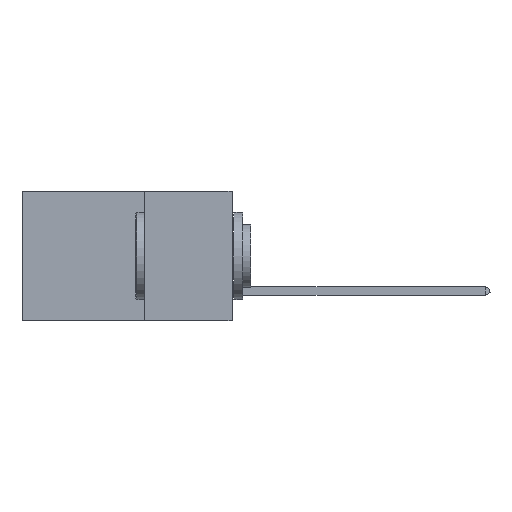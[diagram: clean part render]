
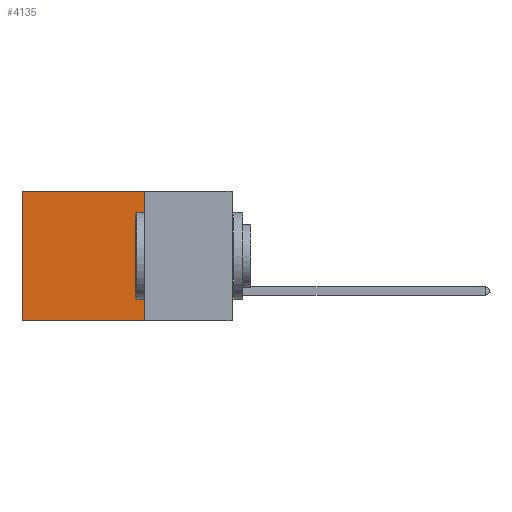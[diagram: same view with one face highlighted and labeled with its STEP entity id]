
A CAD part, left-side view. The second image highlights one B-rep face of the part: STEP entity #4135.
In plain terms, the highlighted planar face has unit normal (-1, 0, 0).
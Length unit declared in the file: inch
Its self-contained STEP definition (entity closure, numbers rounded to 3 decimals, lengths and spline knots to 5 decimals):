
#799 = CARTESIAN_POINT ( 'NONE',  ( 0.2875, 0.6, 0. ) ) ;
#937 = EDGE_CURVE ( 'NONE', #24279, #11036, #28548, .T. ) ;
#951 = LINE ( 'NONE', #27687, #5436 ) ;
#1014 = DIRECTION ( 'NONE',  ( 0., 1., 0. ) ) ;
#2587 = LINE ( 'NONE', #4025, #28113 ) ;
#3701 = EDGE_CURVE ( 'NONE', #27353, #11036, #27990, .T. ) ;
#4025 = CARTESIAN_POINT ( 'NONE',  ( 0.2875, 0.25, 0. ) ) ;
#4135 = ADVANCED_FACE ( 'NONE', ( #23472 ), #27661, .F. ) ;
#5126 = CARTESIAN_POINT ( 'NONE',  ( 0.2875, 0.25, -0.37 ) ) ;
#5436 = VECTOR ( 'NONE', #1014, 39.37008 ) ;
#5672 = ORIENTED_EDGE ( 'NONE', *, *, #3701, .T. ) ;
#6658 = VECTOR ( 'NONE', #14778, 39.37008 ) ;
#7216 = EDGE_CURVE ( 'NONE', #9036, #24279, #2587, .T. ) ;
#7267 = ORIENTED_EDGE ( 'NONE', *, *, #9198, .T. ) ;
#8861 = CARTESIAN_POINT ( 'NONE',  ( 0.2875, 0.6, 0. ) ) ;
#9036 = VERTEX_POINT ( 'NONE', #13981 ) ;
#9198 = EDGE_CURVE ( 'NONE', #9036, #27353, #951, .T. ) ;
#11036 = VERTEX_POINT ( 'NONE', #13730 ) ;
#11047 = ORIENTED_EDGE ( 'NONE', *, *, #937, .F. ) ;
#12531 = DIRECTION ( 'NONE',  ( 0., 0., -1. ) ) ;
#13730 = CARTESIAN_POINT ( 'NONE',  ( 0.2875, 0.6, -0.37 ) ) ;
#13981 = CARTESIAN_POINT ( 'NONE',  ( 0.2875, 0.25, 0. ) ) ;
#14778 = DIRECTION ( 'NONE',  ( 0., 0., -1. ) ) ;
#15271 = ORIENTED_EDGE ( 'NONE', *, *, #7216, .F. ) ;
#15661 = EDGE_LOOP ( 'NONE', ( #5672, #11047, #15271, #7267 ) ) ;
#16283 = DIRECTION ( 'NONE',  ( 0., 0., -1. ) ) ;
#18050 = DIRECTION ( 'NONE',  ( 0., 1., 0. ) ) ;
#20324 = VECTOR ( 'NONE', #18050, 39.37008 ) ;
#23472 = FACE_OUTER_BOUND ( 'NONE', #15661, .T. ) ;
#24019 = AXIS2_PLACEMENT_3D ( 'NONE', #25342, #25434, #16283 ) ;
#24164 = CARTESIAN_POINT ( 'NONE',  ( 0.2875, 0.25, -0.37 ) ) ;
#24279 = VERTEX_POINT ( 'NONE', #24164 ) ;
#25342 = CARTESIAN_POINT ( 'NONE',  ( 0.2875, 0.25, 0. ) ) ;
#25434 = DIRECTION ( 'NONE',  ( 1., 0., 0. ) ) ;
#27353 = VERTEX_POINT ( 'NONE', #8861 ) ;
#27661 = PLANE ( 'NONE',  #24019 ) ;
#27687 = CARTESIAN_POINT ( 'NONE',  ( 0.2875, 0.25, 0. ) ) ;
#27990 = LINE ( 'NONE', #799, #6658 ) ;
#28113 = VECTOR ( 'NONE', #12531, 39.37008 ) ;
#28548 = LINE ( 'NONE', #5126, #20324 ) ;
